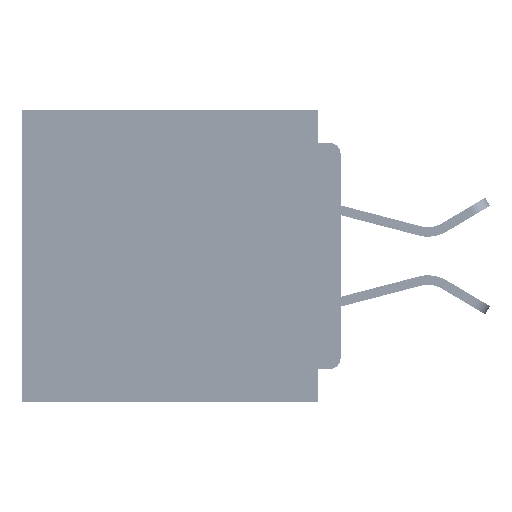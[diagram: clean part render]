
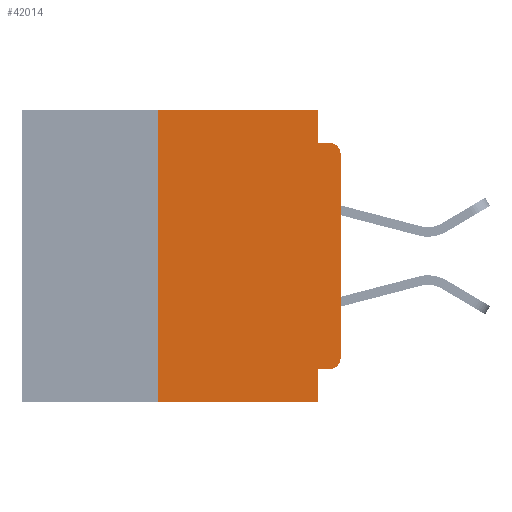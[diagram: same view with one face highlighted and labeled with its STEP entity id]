
A CAD part, left-side view. The second image highlights one B-rep face of the part: STEP entity #42014.
In plain terms, the highlighted planar face has unit normal (-1, 0, 0).
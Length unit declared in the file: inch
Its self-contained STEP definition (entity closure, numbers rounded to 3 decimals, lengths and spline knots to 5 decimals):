
#876 = CARTESIAN_POINT ( 'NONE',  ( 0., 0.015, -0.045 ) ) ;
#1689 = DIRECTION ( 'NONE',  ( 0., 0., -1. ) ) ;
#2373 = AXIS2_PLACEMENT_3D ( 'NONE', #21423, #49612, #25435 ) ;
#2460 = DIRECTION ( 'NONE',  ( 0., 0., 1. ) ) ;
#3978 = CARTESIAN_POINT ( 'NONE',  ( 0., 0.25, 0. ) ) ;
#4169 = VECTOR ( 'NONE', #2460, 39.37008 ) ;
#4733 = ORIENTED_EDGE ( 'NONE', *, *, #49122, .F. ) ;
#5278 = LINE ( 'NONE', #52255, #38832 ) ;
#5441 = LINE ( 'NONE', #22714, #4169 ) ;
#5544 = CARTESIAN_POINT ( 'NONE',  ( 0., 0.031, -0.4 ) ) ;
#5702 = VERTEX_POINT ( 'NONE', #25915 ) ;
#6932 = CARTESIAN_POINT ( 'NONE',  ( 0., 0.031, -0.045 ) ) ;
#7017 = CARTESIAN_POINT ( 'NONE',  ( 0., 0.015, -0.355 ) ) ;
#8022 = DIRECTION ( 'NONE',  ( 0., -1., 0. ) ) ;
#8077 = LINE ( 'NONE', #47731, #49758 ) ;
#9680 = DIRECTION ( 'NONE',  ( 0., 0., -1. ) ) ;
#10733 = EDGE_CURVE ( 'NONE', #23633, #22971, #27068, .T. ) ;
#11138 = EDGE_CURVE ( 'NONE', #5702, #40659, #8077, .T. ) ;
#11827 = VECTOR ( 'NONE', #36757, 39.37008 ) ;
#11983 = VERTEX_POINT ( 'NONE', #45733 ) ;
#12797 = DIRECTION ( 'NONE',  ( -1., 0., 0. ) ) ;
#13056 = EDGE_CURVE ( 'NONE', #46180, #22971, #5278, .T. ) ;
#13206 = EDGE_CURVE ( 'NONE', #18092, #50071, #20536, .T. ) ;
#13389 = VECTOR ( 'NONE', #9680, 39.37008 ) ;
#14256 = VERTEX_POINT ( 'NONE', #45168 ) ;
#15468 = DIRECTION ( 'NONE',  ( 0., -1., 0. ) ) ;
#16309 = EDGE_CURVE ( 'NONE', #50071, #40659, #45555, .T. ) ;
#16367 = DIRECTION ( 'NONE',  ( 0., -1., 0. ) ) ;
#17111 = DIRECTION ( 'NONE',  ( -1., 0., 0. ) ) ;
#18092 = VERTEX_POINT ( 'NONE', #7017 ) ;
#18125 = ORIENTED_EDGE ( 'NONE', *, *, #23183, .F. ) ;
#20536 = LINE ( 'NONE', #29203, #29978 ) ;
#21423 = CARTESIAN_POINT ( 'NONE',  ( 0., 0.437, 0. ) ) ;
#21937 = ORIENTED_EDGE ( 'NONE', *, *, #13206, .F. ) ;
#22714 = CARTESIAN_POINT ( 'NONE',  ( 0., 0.25, -0.4 ) ) ;
#22971 = VERTEX_POINT ( 'NONE', #876 ) ;
#23183 = EDGE_CURVE ( 'NONE', #5702, #42348, #5441, .T. ) ;
#23633 = VERTEX_POINT ( 'NONE', #33790 ) ;
#23694 = EDGE_CURVE ( 'NONE', #11983, #46180, #44596, .T. ) ;
#25435 = DIRECTION ( 'NONE',  ( 0., 0., -1. ) ) ;
#25915 = CARTESIAN_POINT ( 'NONE',  ( 0., 0.25, -0.4 ) ) ;
#27068 = CIRCLE ( 'NONE', #46361, 0.015 ) ;
#28579 = EDGE_CURVE ( 'NONE', #14256, #23633, #43990, .T. ) ;
#28832 = ORIENTED_EDGE ( 'NONE', *, *, #11138, .T. ) ;
#29203 = CARTESIAN_POINT ( 'NONE',  ( 0., 0., -0.355 ) ) ;
#29302 = EDGE_LOOP ( 'NONE', ( #38904, #49626, #52099, #42714, #4733, #18125, #28832, #42098, #21937, #32644 ) ) ;
#29978 = VECTOR ( 'NONE', #49299, 39.37008 ) ;
#32644 = ORIENTED_EDGE ( 'NONE', *, *, #39988, .T. ) ;
#32696 = CARTESIAN_POINT ( 'NONE',  ( 0., 0., 0. ) ) ;
#32927 = LINE ( 'NONE', #51559, #34205 ) ;
#33538 = CARTESIAN_POINT ( 'NONE',  ( 0., 0.031, -0.355 ) ) ;
#33790 = CARTESIAN_POINT ( 'NONE',  ( 0., 0., -0.06 ) ) ;
#34205 = VECTOR ( 'NONE', #15468, 39.37008 ) ;
#36757 = DIRECTION ( 'NONE',  ( 0., 0., 1. ) ) ;
#36966 = CARTESIAN_POINT ( 'NONE',  ( 0., 0.015, -0.34 ) ) ;
#38832 = VECTOR ( 'NONE', #8022, 39.37008 ) ;
#38904 = ORIENTED_EDGE ( 'NONE', *, *, #28579, .T. ) ;
#39800 = CIRCLE ( 'NONE', #50375, 0.015 ) ;
#39988 = EDGE_CURVE ( 'NONE', #18092, #14256, #39800, .T. ) ;
#40659 = VERTEX_POINT ( 'NONE', #40926 ) ;
#40926 = CARTESIAN_POINT ( 'NONE',  ( 0., 0.031, -0.4 ) ) ;
#40988 = DIRECTION ( 'NONE',  ( 0., 0., -1. ) ) ;
#41246 = CARTESIAN_POINT ( 'NONE',  ( 0., 0.015, -0.06 ) ) ;
#41327 = PLANE ( 'NONE',  #2373 ) ;
#42014 = ADVANCED_FACE ( 'NONE', ( #47855 ), #41327, .F. ) ;
#42098 = ORIENTED_EDGE ( 'NONE', *, *, #16309, .F. ) ;
#42348 = VERTEX_POINT ( 'NONE', #3978 ) ;
#42714 = ORIENTED_EDGE ( 'NONE', *, *, #23694, .F. ) ;
#43364 = VECTOR ( 'NONE', #1689, 39.37008 ) ;
#43990 = LINE ( 'NONE', #32696, #11827 ) ;
#44596 = LINE ( 'NONE', #50156, #43364 ) ;
#45168 = CARTESIAN_POINT ( 'NONE',  ( 0., 0., -0.34 ) ) ;
#45315 = DIRECTION ( 'NONE',  ( 0., 0., -1. ) ) ;
#45555 = LINE ( 'NONE', #5544, #13389 ) ;
#45733 = CARTESIAN_POINT ( 'NONE',  ( 0., 0.031, 0. ) ) ;
#46180 = VERTEX_POINT ( 'NONE', #6932 ) ;
#46361 = AXIS2_PLACEMENT_3D ( 'NONE', #41246, #17111, #45315 ) ;
#47731 = CARTESIAN_POINT ( 'NONE',  ( 0., 0.437, -0.4 ) ) ;
#47855 = FACE_OUTER_BOUND ( 'NONE', #29302, .T. ) ;
#49122 = EDGE_CURVE ( 'NONE', #42348, #11983, #32927, .T. ) ;
#49299 = DIRECTION ( 'NONE',  ( 0., 1., 0. ) ) ;
#49612 = DIRECTION ( 'NONE',  ( 1., 0., 0. ) ) ;
#49626 = ORIENTED_EDGE ( 'NONE', *, *, #10733, .T. ) ;
#49758 = VECTOR ( 'NONE', #16367, 39.37008 ) ;
#50071 = VERTEX_POINT ( 'NONE', #33538 ) ;
#50156 = CARTESIAN_POINT ( 'NONE',  ( 0., 0.031, 0. ) ) ;
#50375 = AXIS2_PLACEMENT_3D ( 'NONE', #36966, #12797, #40988 ) ;
#51559 = CARTESIAN_POINT ( 'NONE',  ( 0., 0.437, 0. ) ) ;
#52099 = ORIENTED_EDGE ( 'NONE', *, *, #13056, .F. ) ;
#52255 = CARTESIAN_POINT ( 'NONE',  ( 0., 0., -0.045 ) ) ;
